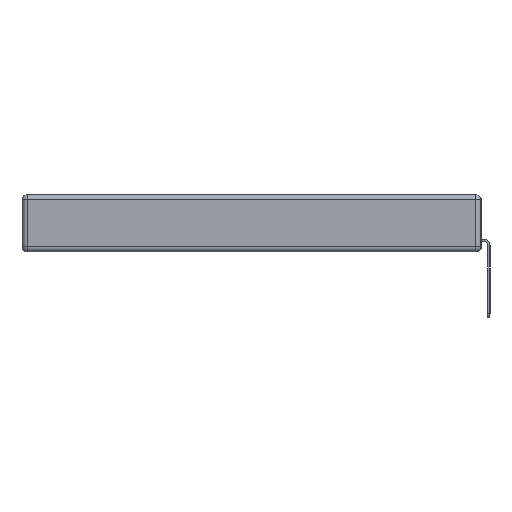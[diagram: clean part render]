
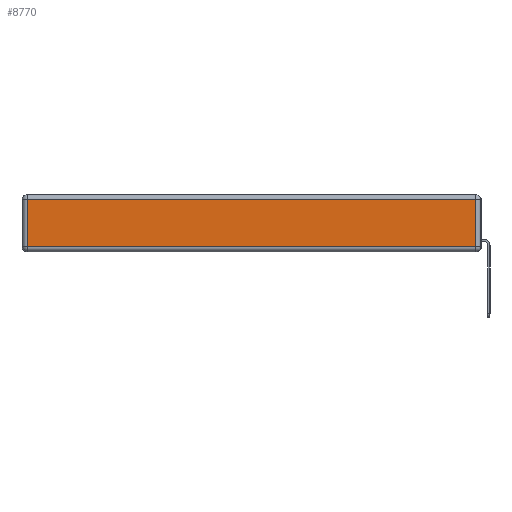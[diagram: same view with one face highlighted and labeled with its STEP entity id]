
A CAD part, left-side view. The second image highlights one B-rep face of the part: STEP entity #8770.
In plain terms, the highlighted planar face has unit normal (-1, 0, 0).
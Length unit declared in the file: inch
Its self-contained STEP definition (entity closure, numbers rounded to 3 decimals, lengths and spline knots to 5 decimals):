
#147 = LINE ( 'NONE', #1472, #2127 ) ;
#678 = LINE ( 'NONE', #5059, #4163 ) ;
#1472 = CARTESIAN_POINT ( 'NONE',  ( 0., 0.03, -0.343 ) ) ;
#1634 = VERTEX_POINT ( 'NONE', #5809 ) ;
#2073 = DIRECTION ( 'NONE',  ( 0., 0., -1. ) ) ;
#2127 = VECTOR ( 'NONE', #9781, 39.37008 ) ;
#2884 = DIRECTION ( 'NONE',  ( 0., 1., 0. ) ) ;
#2910 = DIRECTION ( 'NONE',  ( -1., 0., 0. ) ) ;
#3728 = AXIS2_PLACEMENT_3D ( 'NONE', #13357, #2910, #13426 ) ;
#4163 = VECTOR ( 'NONE', #2884, 39.37008 ) ;
#4360 = ORIENTED_EDGE ( 'NONE', *, *, #9358, .T. ) ;
#4732 = EDGE_CURVE ( 'NONE', #8825, #6198, #147, .T. ) ;
#5059 = CARTESIAN_POINT ( 'NONE',  ( 0., 2.75, -0.03 ) ) ;
#5170 = LINE ( 'NONE', #8542, #8663 ) ;
#5542 = CARTESIAN_POINT ( 'NONE',  ( 0., 2.72, -0.313 ) ) ;
#5809 = CARTESIAN_POINT ( 'NONE',  ( 0., 2.72, -0.03 ) ) ;
#6198 = VERTEX_POINT ( 'NONE', #10827 ) ;
#6396 = CARTESIAN_POINT ( 'NONE',  ( 0., 0., -0.313 ) ) ;
#6692 = LINE ( 'NONE', #6396, #7543 ) ;
#7543 = VECTOR ( 'NONE', #11758, 39.37008 ) ;
#7720 = ORIENTED_EDGE ( 'NONE', *, *, #8059, .T. ) ;
#8059 = EDGE_CURVE ( 'NONE', #9752, #8825, #6692, .T. ) ;
#8261 = EDGE_LOOP ( 'NONE', ( #7720, #9922, #4360, #13705 ) ) ;
#8308 = EDGE_CURVE ( 'NONE', #1634, #9752, #5170, .T. ) ;
#8384 = CARTESIAN_POINT ( 'NONE',  ( 0., 0.03, -0.313 ) ) ;
#8542 = CARTESIAN_POINT ( 'NONE',  ( 0., 2.72, -0.343 ) ) ;
#8663 = VECTOR ( 'NONE', #2073, 39.37008 ) ;
#8770 = ADVANCED_FACE ( 'NONE', ( #9029 ), #12360, .T. ) ;
#8825 = VERTEX_POINT ( 'NONE', #8384 ) ;
#9029 = FACE_OUTER_BOUND ( 'NONE', #8261, .T. ) ;
#9358 = EDGE_CURVE ( 'NONE', #6198, #1634, #678, .T. ) ;
#9752 = VERTEX_POINT ( 'NONE', #5542 ) ;
#9781 = DIRECTION ( 'NONE',  ( 0., 0., 1. ) ) ;
#9922 = ORIENTED_EDGE ( 'NONE', *, *, #4732, .T. ) ;
#10827 = CARTESIAN_POINT ( 'NONE',  ( 0., 0.03, -0.03 ) ) ;
#11758 = DIRECTION ( 'NONE',  ( 0., -1., 0. ) ) ;
#12360 = PLANE ( 'NONE',  #3728 ) ;
#13357 = CARTESIAN_POINT ( 'NONE',  ( 0., 0., -0.343 ) ) ;
#13426 = DIRECTION ( 'NONE',  ( 0., 0., 1. ) ) ;
#13705 = ORIENTED_EDGE ( 'NONE', *, *, #8308, .T. ) ;
